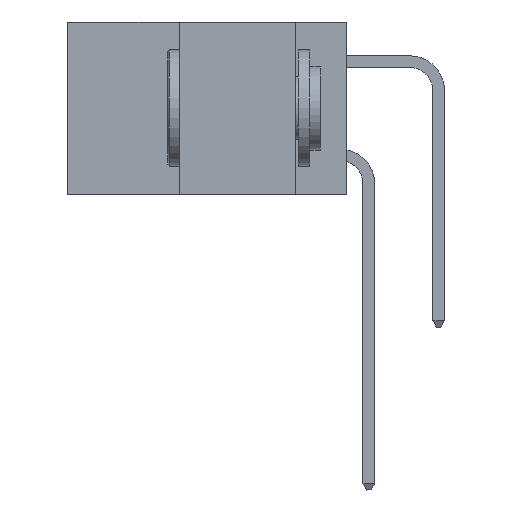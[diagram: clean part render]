
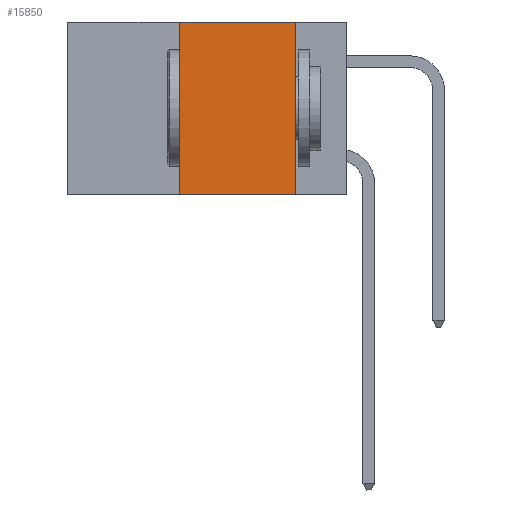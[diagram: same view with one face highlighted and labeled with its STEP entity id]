
A CAD part, left-side view. The second image highlights one B-rep face of the part: STEP entity #15850.
In plain terms, the highlighted planar face has unit normal (-1, 0, 0).
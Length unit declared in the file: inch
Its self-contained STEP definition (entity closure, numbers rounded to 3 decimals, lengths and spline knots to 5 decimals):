
#1296 = EDGE_LOOP ( 'NONE', ( #22573, #8501, #8642, #14922 ) ) ;
#2218 = AXIS2_PLACEMENT_3D ( 'NONE', #10912, #18578, #22285 ) ;
#6331 = VERTEX_POINT ( 'NONE', #11436 ) ;
#6689 = VECTOR ( 'NONE', #15219, 39.37008 ) ;
#7023 = EDGE_CURVE ( 'NONE', #11525, #6331, #17556, .T. ) ;
#7055 = VERTEX_POINT ( 'NONE', #9786 ) ;
#7084 = PLANE ( 'NONE',  #2218 ) ;
#7842 = CARTESIAN_POINT ( 'NONE',  ( 0., 0.36, -0.37 ) ) ;
#8501 = ORIENTED_EDGE ( 'NONE', *, *, #12813, .F. ) ;
#8642 = ORIENTED_EDGE ( 'NONE', *, *, #23262, .F. ) ;
#9786 = CARTESIAN_POINT ( 'NONE',  ( 0., 0.36, 0. ) ) ;
#9990 = CARTESIAN_POINT ( 'NONE',  ( 0., 0.11, 0. ) ) ;
#10912 = CARTESIAN_POINT ( 'NONE',  ( 0., 0.6, 0. ) ) ;
#11190 = EDGE_CURVE ( 'NONE', #14785, #6331, #21592, .T. ) ;
#11436 = CARTESIAN_POINT ( 'NONE',  ( 0., 0.11, -0.37 ) ) ;
#11525 = VERTEX_POINT ( 'NONE', #9990 ) ;
#12813 = EDGE_CURVE ( 'NONE', #7055, #11525, #17349, .T. ) ;
#14506 = VECTOR ( 'NONE', #20330, 39.37008 ) ;
#14785 = VERTEX_POINT ( 'NONE', #7842 ) ;
#14922 = ORIENTED_EDGE ( 'NONE', *, *, #11190, .T. ) ;
#15219 = DIRECTION ( 'NONE',  ( 0., 0., 1. ) ) ;
#15850 = ADVANCED_FACE ( 'NONE', ( #22274 ), #7084, .F. ) ;
#16692 = VECTOR ( 'NONE', #20681, 39.37008 ) ;
#17234 = LINE ( 'NONE', #22812, #6689 ) ;
#17349 = LINE ( 'NONE', #17424, #17980 ) ;
#17424 = CARTESIAN_POINT ( 'NONE',  ( 0., 0.6, 0. ) ) ;
#17556 = LINE ( 'NONE', #22775, #16692 ) ;
#17980 = VECTOR ( 'NONE', #19347, 39.37008 ) ;
#18578 = DIRECTION ( 'NONE',  ( 1., 0., 0. ) ) ;
#19347 = DIRECTION ( 'NONE',  ( 0., -1., 0. ) ) ;
#20330 = DIRECTION ( 'NONE',  ( 0., -1., 0. ) ) ;
#20681 = DIRECTION ( 'NONE',  ( 0., 0., -1. ) ) ;
#21592 = LINE ( 'NONE', #24003, #14506 ) ;
#22274 = FACE_OUTER_BOUND ( 'NONE', #1296, .T. ) ;
#22285 = DIRECTION ( 'NONE',  ( 0., 0., -1. ) ) ;
#22573 = ORIENTED_EDGE ( 'NONE', *, *, #7023, .F. ) ;
#22775 = CARTESIAN_POINT ( 'NONE',  ( 0., 0.11, 0. ) ) ;
#22812 = CARTESIAN_POINT ( 'NONE',  ( 0., 0.36, 0. ) ) ;
#23262 = EDGE_CURVE ( 'NONE', #14785, #7055, #17234, .T. ) ;
#24003 = CARTESIAN_POINT ( 'NONE',  ( 0., 0.6, -0.37 ) ) ;
